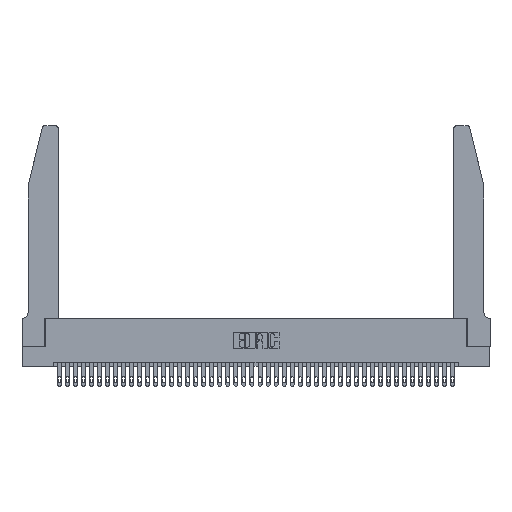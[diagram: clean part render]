
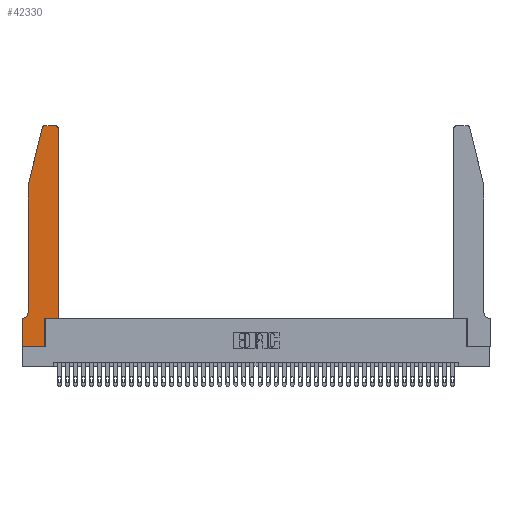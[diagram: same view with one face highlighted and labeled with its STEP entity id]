
A CAD part, top view. The second image highlights one B-rep face of the part: STEP entity #42330.
In plain terms, the highlighted planar face has unit normal (0, 0, 1).
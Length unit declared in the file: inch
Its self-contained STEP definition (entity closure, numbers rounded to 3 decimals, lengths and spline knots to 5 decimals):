
#780 = VECTOR ( 'NONE', #42401, 39.37008 ) ;
#892 = CARTESIAN_POINT ( 'NONE',  ( 0.2865, 0., 0.37 ) ) ;
#1251 = DIRECTION ( 'NONE',  ( 0., 0., 1. ) ) ;
#1550 = CARTESIAN_POINT ( 'NONE',  ( 0., 0., 0.37 ) ) ;
#1878 = DIRECTION ( 'NONE',  ( 1., 0., 0. ) ) ;
#2173 = ORIENTED_EDGE ( 'NONE', *, *, #28412, .T. ) ;
#3032 = DIRECTION ( 'NONE',  ( -1., 0., 0. ) ) ;
#3415 = DIRECTION ( 'NONE',  ( -0.239, -0.971, 0. ) ) ;
#5053 = EDGE_CURVE ( 'NONE', #39820, #40383, #37696, .T. ) ;
#5065 = ORIENTED_EDGE ( 'NONE', *, *, #30261, .T. ) ;
#5552 = LINE ( 'NONE', #6394, #780 ) ;
#5602 = ORIENTED_EDGE ( 'NONE', *, *, #25713, .T. ) ;
#6240 = VECTOR ( 'NONE', #11739, 39.37008 ) ;
#6377 = VECTOR ( 'NONE', #41087, 39.37008 ) ;
#6394 = CARTESIAN_POINT ( 'NONE',  ( 0.0755, 2., 0.37 ) ) ;
#6593 = VERTEX_POINT ( 'NONE', #6736 ) ;
#6736 = CARTESIAN_POINT ( 'NONE',  ( 0., 0.35, 0.37 ) ) ;
#7404 = VERTEX_POINT ( 'NONE', #12584 ) ;
#7818 = PLANE ( 'NONE',  #27116 ) ;
#7835 = ORIENTED_EDGE ( 'NONE', *, *, #37702, .T. ) ;
#7948 = CARTESIAN_POINT ( 'NONE',  ( 0.0055, 0.42, 0.37 ) ) ;
#7996 = CARTESIAN_POINT ( 'NONE',  ( 0.4205, 2.72, 0.37 ) ) ;
#8227 = VECTOR ( 'NONE', #39633, 39.37008 ) ;
#8427 = CARTESIAN_POINT ( 'NONE',  ( 0., 0., 0.37 ) ) ;
#8896 = EDGE_CURVE ( 'NONE', #36609, #23340, #32404, .T. ) ;
#9951 = AXIS2_PLACEMENT_3D ( 'NONE', #7996, #11169, #37178 ) ;
#10309 = LINE ( 'NONE', #8427, #6240 ) ;
#10585 = DIRECTION ( 'NONE',  ( 0., 1., 0. ) ) ;
#11169 = DIRECTION ( 'NONE',  ( 0., 0., 1. ) ) ;
#11255 = EDGE_CURVE ( 'NONE', #20101, #28447, #20292, .T. ) ;
#11653 = CARTESIAN_POINT ( 'NONE',  ( 0., 0., 0.37 ) ) ;
#11739 = DIRECTION ( 'NONE',  ( 0., -1., 0. ) ) ;
#11867 = EDGE_LOOP ( 'NONE', ( #15423, #5602, #5065, #36241, #22087, #7835, #13879, #2173, #14803, #31343, #26856, #14720 ) ) ;
#12584 = CARTESIAN_POINT ( 'NONE',  ( 0.2865, 0.35, 0.37 ) ) ;
#13879 = ORIENTED_EDGE ( 'NONE', *, *, #15893, .T. ) ;
#13951 = VECTOR ( 'NONE', #3415, 39.37008 ) ;
#14720 = ORIENTED_EDGE ( 'NONE', *, *, #32269, .T. ) ;
#14803 = ORIENTED_EDGE ( 'NONE', *, *, #19518, .T. ) ;
#15240 = VECTOR ( 'NONE', #27009, 39.37008 ) ;
#15423 = ORIENTED_EDGE ( 'NONE', *, *, #8896, .T. ) ;
#15893 = EDGE_CURVE ( 'NONE', #6593, #31762, #10309, .T. ) ;
#16351 = CARTESIAN_POINT ( 'NONE',  ( 0.4505, 2.72, 0.37 ) ) ;
#17583 = LINE ( 'NONE', #39272, #13951 ) ;
#18310 = LINE ( 'NONE', #1550, #42654 ) ;
#18445 = CIRCLE ( 'NONE', #9951, 0.03 ) ;
#19518 = EDGE_CURVE ( 'NONE', #42791, #7404, #27148, .T. ) ;
#20101 = VERTEX_POINT ( 'NONE', #27354 ) ;
#20292 = CIRCLE ( 'NONE', #36484, 0.07 ) ;
#21132 = CARTESIAN_POINT ( 'NONE',  ( 0., 0.35, 0.37 ) ) ;
#22087 = ORIENTED_EDGE ( 'NONE', *, *, #11255, .T. ) ;
#22292 = DIRECTION ( 'NONE',  ( 1., 0., 0. ) ) ;
#22648 = LINE ( 'NONE', #35579, #28358 ) ;
#22699 = EDGE_CURVE ( 'NONE', #28281, #20101, #5552, .T. ) ;
#23340 = VERTEX_POINT ( 'NONE', #38331 ) ;
#23656 = CARTESIAN_POINT ( 'NONE',  ( 0.2605, 2.75, 0.37 ) ) ;
#25500 = DIRECTION ( 'NONE',  ( 0., 0., 1. ) ) ;
#25713 = EDGE_CURVE ( 'NONE', #23340, #32788, #35361, .T. ) ;
#26856 = ORIENTED_EDGE ( 'NONE', *, *, #5053, .T. ) ;
#26906 = CARTESIAN_POINT ( 'NONE',  ( 0.25487, 2.72718, 0.37 ) ) ;
#27009 = DIRECTION ( 'NONE',  ( -1., 0., 0. ) ) ;
#27116 = AXIS2_PLACEMENT_3D ( 'NONE', #21132, #1251, #41833 ) ;
#27148 = LINE ( 'NONE', #38698, #39029 ) ;
#27354 = CARTESIAN_POINT ( 'NONE',  ( 0.0755, 0.42, 0.37 ) ) ;
#28281 = VERTEX_POINT ( 'NONE', #31274 ) ;
#28358 = VECTOR ( 'NONE', #3032, 39.37008 ) ;
#28412 = EDGE_CURVE ( 'NONE', #31762, #42791, #18310, .T. ) ;
#28447 = VERTEX_POINT ( 'NONE', #41824 ) ;
#30261 = EDGE_CURVE ( 'NONE', #32788, #28281, #17583, .T. ) ;
#30278 = CARTESIAN_POINT ( 'NONE',  ( 0.4505, 0.35, 0.37 ) ) ;
#30841 = CARTESIAN_POINT ( 'NONE',  ( 0.4505, 0.35, 0.37 ) ) ;
#31230 = LINE ( 'NONE', #30841, #6377 ) ;
#31274 = CARTESIAN_POINT ( 'NONE',  ( 0.0755, 2., 0.37 ) ) ;
#31343 = ORIENTED_EDGE ( 'NONE', *, *, #42243, .T. ) ;
#31762 = VERTEX_POINT ( 'NONE', #11653 ) ;
#32269 = EDGE_CURVE ( 'NONE', #40383, #36609, #18445, .T. ) ;
#32404 = LINE ( 'NONE', #23656, #15240 ) ;
#32788 = VERTEX_POINT ( 'NONE', #26906 ) ;
#32818 = CARTESIAN_POINT ( 'NONE',  ( 0.4205, 2.75, 0.37 ) ) ;
#35361 = CIRCLE ( 'NONE', #40281, 0.03 ) ;
#35579 = CARTESIAN_POINT ( 'NONE',  ( 0.0755, 0.35, 0.37 ) ) ;
#36241 = ORIENTED_EDGE ( 'NONE', *, *, #22699, .T. ) ;
#36484 = AXIS2_PLACEMENT_3D ( 'NONE', #7948, #38182, #38917 ) ;
#36609 = VERTEX_POINT ( 'NONE', #32818 ) ;
#37178 = DIRECTION ( 'NONE',  ( 1., 0., 0. ) ) ;
#37696 = LINE ( 'NONE', #30278, #8227 ) ;
#37702 = EDGE_CURVE ( 'NONE', #28447, #6593, #22648, .T. ) ;
#38182 = DIRECTION ( 'NONE',  ( 0., 0., -1. ) ) ;
#38331 = CARTESIAN_POINT ( 'NONE',  ( 0.284, 2.75, 0.37 ) ) ;
#38698 = CARTESIAN_POINT ( 'NONE',  ( 0.2865, 0.35, 0.37 ) ) ;
#38917 = DIRECTION ( 'NONE',  ( -1., 0., 0. ) ) ;
#39029 = VECTOR ( 'NONE', #10585, 39.37008 ) ;
#39272 = CARTESIAN_POINT ( 'NONE',  ( 0.0755, 2., 0.37 ) ) ;
#39633 = DIRECTION ( 'NONE',  ( 0., 1., 0. ) ) ;
#39820 = VERTEX_POINT ( 'NONE', #40078 ) ;
#40078 = CARTESIAN_POINT ( 'NONE',  ( 0.4505, 0.35, 0.37 ) ) ;
#40281 = AXIS2_PLACEMENT_3D ( 'NONE', #42517, #25500, #22292 ) ;
#40383 = VERTEX_POINT ( 'NONE', #16351 ) ;
#41087 = DIRECTION ( 'NONE',  ( 1., 0., 0. ) ) ;
#41824 = CARTESIAN_POINT ( 'NONE',  ( 0.0055, 0.35, 0.37 ) ) ;
#41833 = DIRECTION ( 'NONE',  ( 1., 0., 0. ) ) ;
#42243 = EDGE_CURVE ( 'NONE', #7404, #39820, #31230, .T. ) ;
#42330 = ADVANCED_FACE ( 'NONE', ( #42598 ), #7818, .T. ) ;
#42401 = DIRECTION ( 'NONE',  ( 0., -1., 0. ) ) ;
#42517 = CARTESIAN_POINT ( 'NONE',  ( 0.284, 2.72, 0.37 ) ) ;
#42598 = FACE_OUTER_BOUND ( 'NONE', #11867, .T. ) ;
#42654 = VECTOR ( 'NONE', #1878, 39.37008 ) ;
#42791 = VERTEX_POINT ( 'NONE', #892 ) ;
